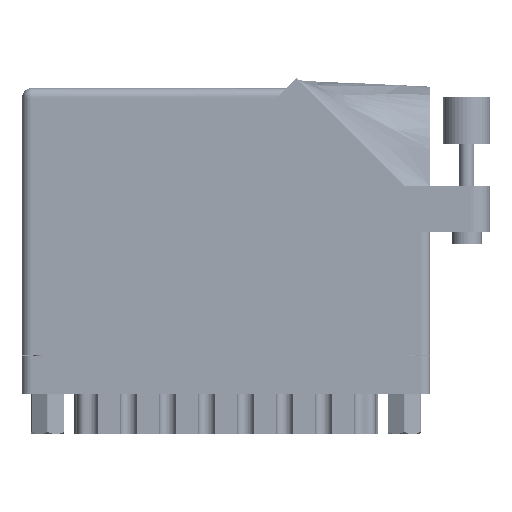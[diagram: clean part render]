
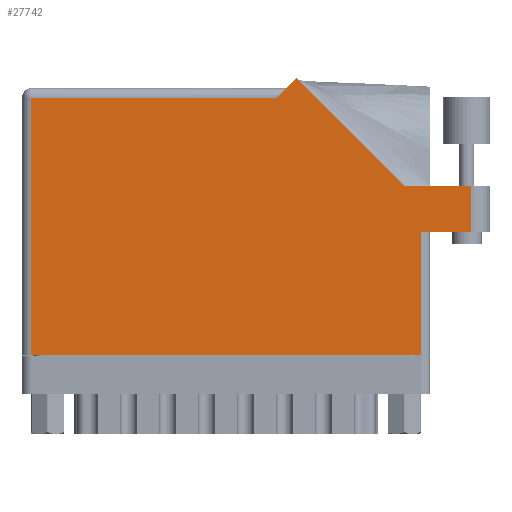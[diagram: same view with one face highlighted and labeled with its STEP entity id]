
A CAD part, front view. The second image highlights one B-rep face of the part: STEP entity #27742.
In plain terms, the highlighted face is planar.
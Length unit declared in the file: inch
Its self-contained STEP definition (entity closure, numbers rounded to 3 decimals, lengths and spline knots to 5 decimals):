
#64 = DIRECTION ( 'NONE',  ( 0., 1., 0. ) ) ;
#801 = ORIENTED_EDGE ( 'NONE', *, *, #47796, .T. ) ;
#3144 = VERTEX_POINT ( 'NONE', #47776 ) ;
#5749 = DIRECTION ( 'NONE',  ( -0.707, -0.707, 0. ) ) ;
#6871 = VERTEX_POINT ( 'NONE', #22221 ) ;
#8649 = LINE ( 'NONE', #58579, #68881 ) ;
#8692 = CARTESIAN_POINT ( 'NONE',  ( 2.993, 0.815, 0. ) ) ;
#9337 = DIRECTION ( 'NONE',  ( 0., -1., 0. ) ) ;
#9937 = EDGE_CURVE ( 'NONE', #56053, #3144, #14304, .T. ) ;
#10052 = EDGE_CURVE ( 'NONE', #42726, #85530, #31891, .T. ) ;
#11086 = CARTESIAN_POINT ( 'NONE',  ( 1.696, 1.713, 0. ) ) ;
#13225 = ORIENTED_EDGE ( 'NONE', *, *, #10052, .T. ) ;
#14304 = LINE ( 'NONE', #32089, #51668 ) ;
#15556 = AXIS2_PLACEMENT_3D ( 'NONE', #84887, #32559, #19559 ) ;
#16903 = VERTEX_POINT ( 'NONE', #82244 ) ;
#17270 = ORIENTED_EDGE ( 'NONE', *, *, #9937, .T. ) ;
#17929 = EDGE_CURVE ( 'NONE', #31703, #56053, #41894, .T. ) ;
#18885 = VECTOR ( 'NONE', #48091, 39.37008 ) ;
#19559 = DIRECTION ( 'NONE',  ( -1., 0., 0. ) ) ;
#20965 = LINE ( 'NONE', #61977, #18885 ) ;
#21231 = LINE ( 'NONE', #29221, #44014 ) ;
#22221 = CARTESIAN_POINT ( 'NONE',  ( 1.82871, 1.84571, 0. ) ) ;
#23515 = CARTESIAN_POINT ( 'NONE',  ( 0.062, 0., 0. ) ) ;
#26251 = CARTESIAN_POINT ( 'NONE',  ( 3.118, 1.122, 0. ) ) ;
#27742 = ADVANCED_FACE ( 'NONE', ( #67525 ), #38946, .F. ) ;
#28798 = VECTOR ( 'NONE', #64, 39.37008 ) ;
#29221 = CARTESIAN_POINT ( 'NONE',  ( 2.718, 0.815, 0. ) ) ;
#31249 = CARTESIAN_POINT ( 'NONE',  ( 0., 1.713, 0. ) ) ;
#31407 = ORIENTED_EDGE ( 'NONE', *, *, #67239, .T. ) ;
#31703 = VERTEX_POINT ( 'NONE', #23515 ) ;
#31891 = LINE ( 'NONE', #31249, #55831 ) ;
#32089 = CARTESIAN_POINT ( 'NONE',  ( 2.656, 0.815, 0. ) ) ;
#32559 = DIRECTION ( 'NONE',  ( 0., 0., -1. ) ) ;
#32664 = EDGE_CURVE ( 'NONE', #77512, #75350, #64084, .T. ) ;
#32872 = DIRECTION ( 'NONE',  ( -1., 0., 0. ) ) ;
#33737 = CARTESIAN_POINT ( 'NONE',  ( 0.062, 1.713, 0. ) ) ;
#34594 = ORIENTED_EDGE ( 'NONE', *, *, #76525, .T. ) ;
#35720 = LINE ( 'NONE', #26251, #37807 ) ;
#37807 = VECTOR ( 'NONE', #32872, 39.37008 ) ;
#38166 = LINE ( 'NONE', #78180, #57917 ) ;
#38203 = DIRECTION ( 'NONE',  ( 0., 1., 0. ) ) ;
#38946 = PLANE ( 'NONE',  #15556 ) ;
#39780 = CARTESIAN_POINT ( 'NONE',  ( 2.993, 1.122, 0. ) ) ;
#41894 = LINE ( 'NONE', #73907, #53298 ) ;
#42726 = VERTEX_POINT ( 'NONE', #11086 ) ;
#44014 = VECTOR ( 'NONE', #82667, 39.37008 ) ;
#47776 = CARTESIAN_POINT ( 'NONE',  ( 2.656, 0.815, 0. ) ) ;
#47796 = EDGE_CURVE ( 'NONE', #85530, #31703, #38166, .T. ) ;
#48091 = DIRECTION ( 'NONE',  ( -0.707, 0.707, 0. ) ) ;
#49449 = ORIENTED_EDGE ( 'NONE', *, *, #82181, .T. ) ;
#51668 = VECTOR ( 'NONE', #38203, 39.37008 ) ;
#53298 = VECTOR ( 'NONE', #60819, 39.37008 ) ;
#54702 = ORIENTED_EDGE ( 'NONE', *, *, #81410, .T. ) ;
#55831 = VECTOR ( 'NONE', #64900, 39.37008 ) ;
#55995 = EDGE_LOOP ( 'NONE', ( #54702, #72837, #34594, #31407, #49449, #13225, #801, #58562, #17270 ) ) ;
#56053 = VERTEX_POINT ( 'NONE', #58717 ) ;
#57917 = VECTOR ( 'NONE', #9337, 39.37008 ) ;
#58562 = ORIENTED_EDGE ( 'NONE', *, *, #17929, .T. ) ;
#58579 = CARTESIAN_POINT ( 'NONE',  ( 1.758, 1.775, 0. ) ) ;
#58717 = CARTESIAN_POINT ( 'NONE',  ( 2.656, 0., 0. ) ) ;
#60819 = DIRECTION ( 'NONE',  ( 1., 0., 0. ) ) ;
#61977 = CARTESIAN_POINT ( 'NONE',  ( 2.55242, 1.122, 0. ) ) ;
#64084 = LINE ( 'NONE', #39780, #28798 ) ;
#64900 = DIRECTION ( 'NONE',  ( -1., 0., 0. ) ) ;
#67239 = EDGE_CURVE ( 'NONE', #16903, #6871, #20965, .T. ) ;
#67525 = FACE_OUTER_BOUND ( 'NONE', #55995, .T. ) ;
#68881 = VECTOR ( 'NONE', #5749, 39.37008 ) ;
#72837 = ORIENTED_EDGE ( 'NONE', *, *, #32664, .T. ) ;
#73907 = CARTESIAN_POINT ( 'NONE',  ( 0., 0., 0. ) ) ;
#75350 = VERTEX_POINT ( 'NONE', #85693 ) ;
#76525 = EDGE_CURVE ( 'NONE', #75350, #16903, #35720, .T. ) ;
#77512 = VERTEX_POINT ( 'NONE', #8692 ) ;
#78180 = CARTESIAN_POINT ( 'NONE',  ( 0.062, 0., 0. ) ) ;
#81410 = EDGE_CURVE ( 'NONE', #3144, #77512, #21231, .T. ) ;
#82181 = EDGE_CURVE ( 'NONE', #6871, #42726, #8649, .T. ) ;
#82244 = CARTESIAN_POINT ( 'NONE',  ( 2.55242, 1.122, 0. ) ) ;
#82667 = DIRECTION ( 'NONE',  ( 1., 0., 0. ) ) ;
#84887 = CARTESIAN_POINT ( 'NONE',  ( 0., 1.775, 0. ) ) ;
#85530 = VERTEX_POINT ( 'NONE', #33737 ) ;
#85693 = CARTESIAN_POINT ( 'NONE',  ( 2.993, 1.122, 0. ) ) ;
